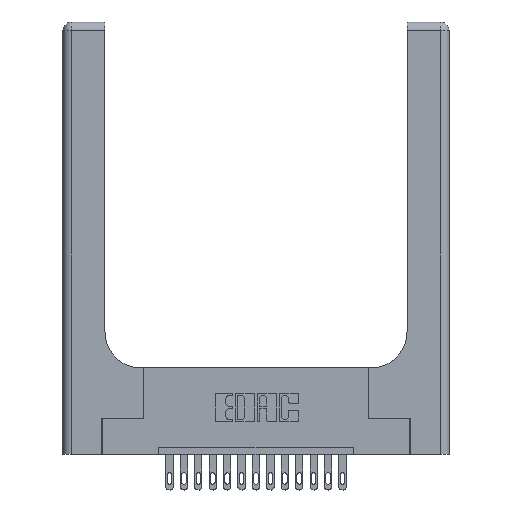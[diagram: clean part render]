
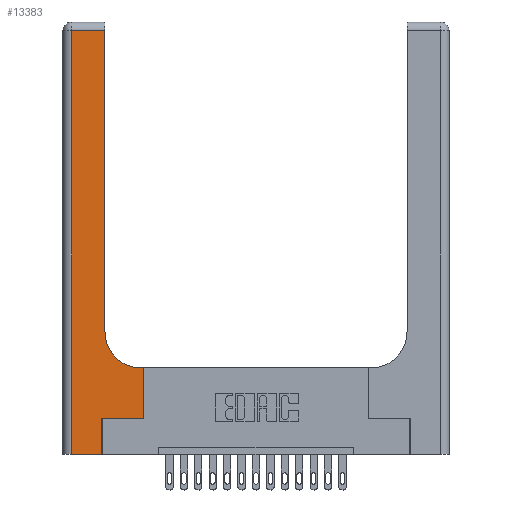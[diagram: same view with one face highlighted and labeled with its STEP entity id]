
A CAD part, top view. The second image highlights one B-rep face of the part: STEP entity #13383.
In plain terms, the highlighted planar face has unit normal (0, 0, 1).
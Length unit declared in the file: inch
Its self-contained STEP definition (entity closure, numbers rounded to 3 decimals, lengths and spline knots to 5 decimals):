
#1065 = CIRCLE ( 'NONE', #8773, 0.25 ) ;
#1206 = EDGE_CURVE ( 'NONE', #12088, #2393, #11343, .T. ) ;
#1244 = CARTESIAN_POINT ( 'NONE',  ( 0., 2.94, 0.37 ) ) ;
#1256 = DIRECTION ( 'NONE',  ( 1., 0., 0. ) ) ;
#1339 = CARTESIAN_POINT ( 'NONE',  ( 0.06, 2.94, 0.37 ) ) ;
#1450 = ORIENTED_EDGE ( 'NONE', *, *, #1206, .T. ) ;
#2393 = VERTEX_POINT ( 'NONE', #6672 ) ;
#2498 = EDGE_LOOP ( 'NONE', ( #6716, #17839, #15893, #14065, #1450, #18315, #14581, #12446, #9587 ) ) ;
#2698 = DIRECTION ( 'NONE',  ( -1., 0., 0. ) ) ;
#3351 = VECTOR ( 'NONE', #18173, 39.37008 ) ;
#3425 = CARTESIAN_POINT ( 'NONE',  ( 0.5585, 0.6, 0.37 ) ) ;
#3631 = CARTESIAN_POINT ( 'NONE',  ( 0.5585, 0.25, 0.37 ) ) ;
#3656 = VECTOR ( 'NONE', #5140, 39.37008 ) ;
#3700 = CARTESIAN_POINT ( 'NONE',  ( 0.269, 0.25, 0.37 ) ) ;
#3768 = VERTEX_POINT ( 'NONE', #9668 ) ;
#3871 = CARTESIAN_POINT ( 'NONE',  ( 0.2915, 0.85, 0.37 ) ) ;
#3970 = VECTOR ( 'NONE', #9586, 39.37008 ) ;
#4090 = EDGE_CURVE ( 'NONE', #5342, #6021, #17237, .T. ) ;
#4144 = CARTESIAN_POINT ( 'NONE',  ( 0.06, 0., 0.37 ) ) ;
#4154 = VECTOR ( 'NONE', #13779, 39.37008 ) ;
#4302 = CARTESIAN_POINT ( 'NONE',  ( 0.269, 0., 0.37 ) ) ;
#4835 = EDGE_CURVE ( 'NONE', #9512, #12087, #1065, .T. ) ;
#5140 = DIRECTION ( 'NONE',  ( 0., 1., 0. ) ) ;
#5342 = VERTEX_POINT ( 'NONE', #12893 ) ;
#5526 = FACE_OUTER_BOUND ( 'NONE', #2498, .T. ) ;
#5537 = DIRECTION ( 'NONE',  ( 0., 0., -1. ) ) ;
#6021 = VERTEX_POINT ( 'NONE', #3425 ) ;
#6193 = LINE ( 'NONE', #3700, #3970 ) ;
#6218 = LINE ( 'NONE', #1244, #15795 ) ;
#6239 = LINE ( 'NONE', #11930, #9214 ) ;
#6451 = DIRECTION ( 'NONE',  ( 1., 0., 0. ) ) ;
#6466 = CARTESIAN_POINT ( 'NONE',  ( 0.2915, 0.6, 0.37 ) ) ;
#6672 = CARTESIAN_POINT ( 'NONE',  ( 0.269, 0.25, 0.37 ) ) ;
#6716 = ORIENTED_EDGE ( 'NONE', *, *, #18041, .T. ) ;
#6720 = VECTOR ( 'NONE', #6451, 39.37008 ) ;
#6871 = CARTESIAN_POINT ( 'NONE',  ( 0.5415, 0.85, 0.37 ) ) ;
#6962 = VECTOR ( 'NONE', #9436, 39.37008 ) ;
#7279 = VERTEX_POINT ( 'NONE', #4144 ) ;
#7338 = DIRECTION ( 'NONE',  ( 0., -1., 0. ) ) ;
#7793 = VERTEX_POINT ( 'NONE', #1339 ) ;
#8431 = CARTESIAN_POINT ( 'NONE',  ( 0., 3., 0.37 ) ) ;
#8773 = AXIS2_PLACEMENT_3D ( 'NONE', #6871, #5537, #1256 ) ;
#9019 = LINE ( 'NONE', #16885, #6962 ) ;
#9214 = VECTOR ( 'NONE', #7338, 39.37008 ) ;
#9436 = DIRECTION ( 'NONE',  ( 0., 1., 0. ) ) ;
#9446 = AXIS2_PLACEMENT_3D ( 'NONE', #8431, #18620, #2698 ) ;
#9512 = VERTEX_POINT ( 'NONE', #14072 ) ;
#9586 = DIRECTION ( 'NONE',  ( 1., 0., 0. ) ) ;
#9587 = ORIENTED_EDGE ( 'NONE', *, *, #4835, .T. ) ;
#9668 = CARTESIAN_POINT ( 'NONE',  ( 0.2915, 2.94, 0.37 ) ) ;
#9816 = CARTESIAN_POINT ( 'NONE',  ( 0.269, 0., 0.37 ) ) ;
#10011 = DIRECTION ( 'NONE',  ( -1., 0., 0. ) ) ;
#10839 = EDGE_CURVE ( 'NONE', #3768, #7793, #6218, .T. ) ;
#10902 = EDGE_CURVE ( 'NONE', #7793, #7279, #6239, .T. ) ;
#11343 = LINE ( 'NONE', #4302, #3656 ) ;
#11930 = CARTESIAN_POINT ( 'NONE',  ( 0.06, 3., 0.37 ) ) ;
#12087 = VERTEX_POINT ( 'NONE', #3871 ) ;
#12088 = VERTEX_POINT ( 'NONE', #9816 ) ;
#12446 = ORIENTED_EDGE ( 'NONE', *, *, #14406, .T. ) ;
#12813 = PLANE ( 'NONE',  #9446 ) ;
#12893 = CARTESIAN_POINT ( 'NONE',  ( 0.5585, 0.25, 0.37 ) ) ;
#13124 = EDGE_CURVE ( 'NONE', #2393, #5342, #6193, .T. ) ;
#13383 = ADVANCED_FACE ( 'NONE', ( #5526 ), #12813, .F. ) ;
#13424 = LINE ( 'NONE', #6466, #4154 ) ;
#13779 = DIRECTION ( 'NONE',  ( -1., 0., 0. ) ) ;
#13894 = CARTESIAN_POINT ( 'NONE',  ( 0., 0., 0.37 ) ) ;
#14065 = ORIENTED_EDGE ( 'NONE', *, *, #17373, .T. ) ;
#14072 = CARTESIAN_POINT ( 'NONE',  ( 0.5415, 0.6, 0.37 ) ) ;
#14406 = EDGE_CURVE ( 'NONE', #6021, #9512, #13424, .T. ) ;
#14581 = ORIENTED_EDGE ( 'NONE', *, *, #4090, .T. ) ;
#15795 = VECTOR ( 'NONE', #10011, 39.37008 ) ;
#15893 = ORIENTED_EDGE ( 'NONE', *, *, #10902, .T. ) ;
#16885 = CARTESIAN_POINT ( 'NONE',  ( 0.2915, 3., 0.37 ) ) ;
#17237 = LINE ( 'NONE', #3631, #3351 ) ;
#17373 = EDGE_CURVE ( 'NONE', #7279, #12088, #18337, .T. ) ;
#17839 = ORIENTED_EDGE ( 'NONE', *, *, #10839, .T. ) ;
#18041 = EDGE_CURVE ( 'NONE', #12087, #3768, #9019, .T. ) ;
#18173 = DIRECTION ( 'NONE',  ( 0., 1., 0. ) ) ;
#18315 = ORIENTED_EDGE ( 'NONE', *, *, #13124, .T. ) ;
#18337 = LINE ( 'NONE', #13894, #6720 ) ;
#18620 = DIRECTION ( 'NONE',  ( 0., 0., -1. ) ) ;
